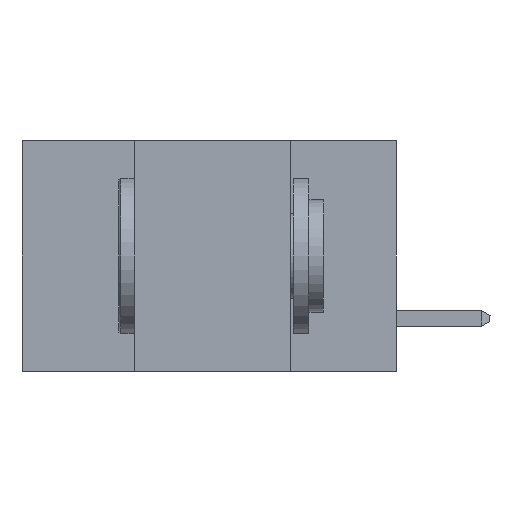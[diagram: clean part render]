
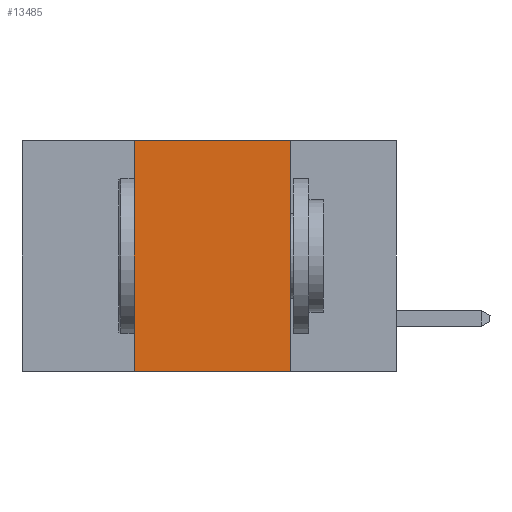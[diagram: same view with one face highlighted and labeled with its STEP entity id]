
A CAD part, left-side view. The second image highlights one B-rep face of the part: STEP entity #13485.
In plain terms, the highlighted planar face has unit normal (-1, 0, 0).
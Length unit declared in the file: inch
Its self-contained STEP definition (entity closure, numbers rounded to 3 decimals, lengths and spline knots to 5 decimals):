
#768 = CARTESIAN_POINT ( 'NONE',  ( 0., 0.17, -0.37 ) ) ;
#843 = VECTOR ( 'NONE', #18740, 39.37008 ) ;
#1253 = DIRECTION ( 'NONE',  ( 0., 0., -1. ) ) ;
#1336 = LINE ( 'NONE', #11670, #843 ) ;
#1534 = LINE ( 'NONE', #14703, #6118 ) ;
#1765 = EDGE_CURVE ( 'NONE', #18797, #13309, #10843, .T. ) ;
#2645 = VECTOR ( 'NONE', #19522, 39.37008 ) ;
#3653 = CARTESIAN_POINT ( 'NONE',  ( 0., 0.42, 0. ) ) ;
#3689 = LINE ( 'NONE', #768, #8734 ) ;
#3859 = EDGE_CURVE ( 'NONE', #13309, #6631, #1336, .T. ) ;
#3957 = CARTESIAN_POINT ( 'NONE',  ( 0., 0.17, 0. ) ) ;
#5413 = DIRECTION ( 'NONE',  ( 0., -1., 0. ) ) ;
#5489 = ORIENTED_EDGE ( 'NONE', *, *, #6967, .F. ) ;
#5533 = PLANE ( 'NONE',  #13329 ) ;
#6118 = VECTOR ( 'NONE', #5413, 39.37008 ) ;
#6402 = EDGE_LOOP ( 'NONE', ( #5489, #6506, #8833, #10039 ) ) ;
#6506 = ORIENTED_EDGE ( 'NONE', *, *, #3859, .F. ) ;
#6631 = VERTEX_POINT ( 'NONE', #3957 ) ;
#6967 = EDGE_CURVE ( 'NONE', #6631, #9596, #3689, .T. ) ;
#7661 = FACE_OUTER_BOUND ( 'NONE', #6402, .T. ) ;
#8621 = DIRECTION ( 'NONE',  ( 1., 0., 0. ) ) ;
#8734 = VECTOR ( 'NONE', #1253, 39.37008 ) ;
#8833 = ORIENTED_EDGE ( 'NONE', *, *, #1765, .F. ) ;
#9596 = VERTEX_POINT ( 'NONE', #14240 ) ;
#10039 = ORIENTED_EDGE ( 'NONE', *, *, #18561, .T. ) ;
#10843 = LINE ( 'NONE', #19617, #2645 ) ;
#11670 = CARTESIAN_POINT ( 'NONE',  ( 0., 0.6, 0. ) ) ;
#13309 = VERTEX_POINT ( 'NONE', #3653 ) ;
#13329 = AXIS2_PLACEMENT_3D ( 'NONE', #16289, #8621, #19225 ) ;
#13485 = ADVANCED_FACE ( 'NONE', ( #7661 ), #5533, .F. ) ;
#13709 = CARTESIAN_POINT ( 'NONE',  ( 0., 0.42, -0.37 ) ) ;
#14240 = CARTESIAN_POINT ( 'NONE',  ( 0., 0.17, -0.37 ) ) ;
#14703 = CARTESIAN_POINT ( 'NONE',  ( 0., 0.6, -0.37 ) ) ;
#16289 = CARTESIAN_POINT ( 'NONE',  ( 0., 0.6, 0. ) ) ;
#18561 = EDGE_CURVE ( 'NONE', #18797, #9596, #1534, .T. ) ;
#18740 = DIRECTION ( 'NONE',  ( 0., -1., 0. ) ) ;
#18797 = VERTEX_POINT ( 'NONE', #13709 ) ;
#19225 = DIRECTION ( 'NONE',  ( 0., 0., -1. ) ) ;
#19522 = DIRECTION ( 'NONE',  ( 0., 0., 1. ) ) ;
#19617 = CARTESIAN_POINT ( 'NONE',  ( 0., 0.42, -0.37 ) ) ;
